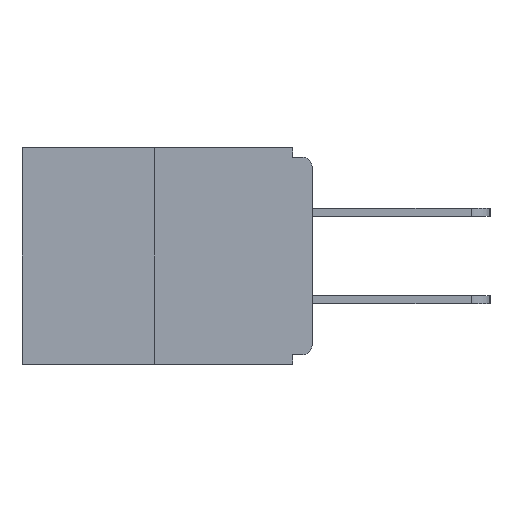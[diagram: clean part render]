
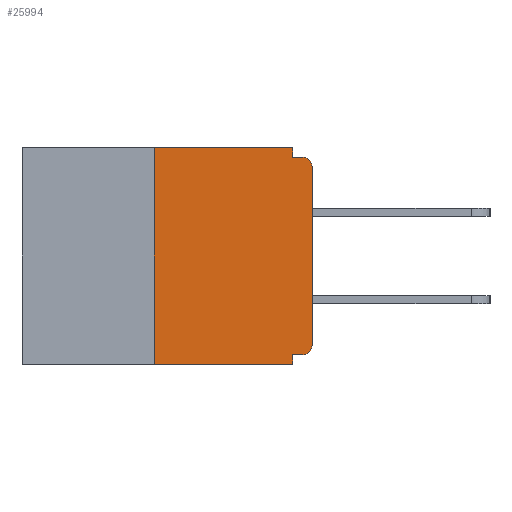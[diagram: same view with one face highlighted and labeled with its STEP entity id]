
A CAD part, left-side view. The second image highlights one B-rep face of the part: STEP entity #25994.
In plain terms, the highlighted planar face has unit normal (-1, 0, 0).
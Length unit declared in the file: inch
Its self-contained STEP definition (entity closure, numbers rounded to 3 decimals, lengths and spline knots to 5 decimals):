
#137 = DIRECTION ( 'NONE',  ( 0., 1., 0. ) ) ;
#1248 = LINE ( 'NONE', #21852, #16392 ) ;
#1658 = LINE ( 'NONE', #13782, #18388 ) ;
#2026 = LINE ( 'NONE', #14864, #24063 ) ;
#2213 = CARTESIAN_POINT ( 'NONE',  ( 0., 0., -0.328 ) ) ;
#2914 = DIRECTION ( 'NONE',  ( -1., 0., 0. ) ) ;
#3069 = DIRECTION ( 'NONE',  ( 0., 0., -1. ) ) ;
#3260 = CARTESIAN_POINT ( 'NONE',  ( 0., 0.031, -0.328 ) ) ;
#3447 = DIRECTION ( 'NONE',  ( 0., 0., -1. ) ) ;
#3623 = VECTOR ( 'NONE', #137, 39.37008 ) ;
#4881 = CARTESIAN_POINT ( 'NONE',  ( 0., 0.015, -0.313 ) ) ;
#4946 = CARTESIAN_POINT ( 'NONE',  ( 0., 0.46, 0. ) ) ;
#5291 = LINE ( 'NONE', #13303, #10782 ) ;
#5676 = CARTESIAN_POINT ( 'NONE',  ( 0., 0., -0.015 ) ) ;
#6066 = ORIENTED_EDGE ( 'NONE', *, *, #24553, .T. ) ;
#6385 = ORIENTED_EDGE ( 'NONE', *, *, #16559, .F. ) ;
#6531 = VERTEX_POINT ( 'NONE', #26326 ) ;
#6546 = ORIENTED_EDGE ( 'NONE', *, *, #11780, .F. ) ;
#6860 = EDGE_CURVE ( 'NONE', #15650, #23880, #1248, .T. ) ;
#7014 = ORIENTED_EDGE ( 'NONE', *, *, #19091, .T. ) ;
#7026 = VECTOR ( 'NONE', #22215, 39.37008 ) ;
#7319 = VERTEX_POINT ( 'NONE', #23950 ) ;
#7407 = PLANE ( 'NONE',  #8398 ) ;
#7681 = DIRECTION ( 'NONE',  ( 0., -1., 0. ) ) ;
#8398 = AXIS2_PLACEMENT_3D ( 'NONE', #9449, #11152, #25750 ) ;
#8469 = VERTEX_POINT ( 'NONE', #24242 ) ;
#8923 = VERTEX_POINT ( 'NONE', #3260 ) ;
#9086 = LINE ( 'NONE', #2213, #3623 ) ;
#9126 = DIRECTION ( 'NONE',  ( 0., 0., -1. ) ) ;
#9228 = ORIENTED_EDGE ( 'NONE', *, *, #6860, .T. ) ;
#9256 = LINE ( 'NONE', #5676, #7026 ) ;
#9421 = LINE ( 'NONE', #22024, #20637 ) ;
#9449 = CARTESIAN_POINT ( 'NONE',  ( 0., 0.46, 0. ) ) ;
#9699 = CIRCLE ( 'NONE', #12723, 0.015 ) ;
#9724 = VECTOR ( 'NONE', #21077, 39.37008 ) ;
#10782 = VECTOR ( 'NONE', #3069, 39.37008 ) ;
#11035 = CARTESIAN_POINT ( 'NONE',  ( 0., 0., -0.03 ) ) ;
#11149 = ORIENTED_EDGE ( 'NONE', *, *, #22864, .T. ) ;
#11152 = DIRECTION ( 'NONE',  ( 1., 0., 0. ) ) ;
#11780 = EDGE_CURVE ( 'NONE', #19613, #20787, #2026, .T. ) ;
#12723 = AXIS2_PLACEMENT_3D ( 'NONE', #14050, #15920, #3447 ) ;
#13303 = CARTESIAN_POINT ( 'NONE',  ( 0., 0.031, -0.343 ) ) ;
#13337 = VERTEX_POINT ( 'NONE', #16639 ) ;
#13609 = CARTESIAN_POINT ( 'NONE',  ( 0., 0.031, 0. ) ) ;
#13782 = CARTESIAN_POINT ( 'NONE',  ( 0., 0.031, 0. ) ) ;
#14050 = CARTESIAN_POINT ( 'NONE',  ( 0., 0.015, -0.03 ) ) ;
#14051 = ORIENTED_EDGE ( 'NONE', *, *, #15014, .F. ) ;
#14308 = ORIENTED_EDGE ( 'NONE', *, *, #18719, .F. ) ;
#14864 = CARTESIAN_POINT ( 'NONE',  ( 0., 0.25, 0. ) ) ;
#15014 = EDGE_CURVE ( 'NONE', #8923, #7319, #5291, .T. ) ;
#15650 = VERTEX_POINT ( 'NONE', #23675 ) ;
#15832 = ORIENTED_EDGE ( 'NONE', *, *, #21000, .F. ) ;
#15837 = ORIENTED_EDGE ( 'NONE', *, *, #25597, .F. ) ;
#15920 = DIRECTION ( 'NONE',  ( -1., 0., 0. ) ) ;
#16281 = CARTESIAN_POINT ( 'NONE',  ( 0., 0.25, 0. ) ) ;
#16392 = VECTOR ( 'NONE', #26255, 39.37008 ) ;
#16524 = EDGE_LOOP ( 'NONE', ( #14308, #6546, #6066, #14051, #6385, #11149, #9228, #7014, #15832, #15837 ) ) ;
#16559 = EDGE_CURVE ( 'NONE', #8469, #8923, #9086, .T. ) ;
#16639 = CARTESIAN_POINT ( 'NONE',  ( 0., 0.031, -0.015 ) ) ;
#18376 = DIRECTION ( 'NONE',  ( 0., 0., -1. ) ) ;
#18388 = VECTOR ( 'NONE', #18376, 39.37008 ) ;
#18719 = EDGE_CURVE ( 'NONE', #20787, #19657, #21829, .T. ) ;
#18951 = DIRECTION ( 'NONE',  ( 0., 0., 1. ) ) ;
#19091 = EDGE_CURVE ( 'NONE', #23880, #6531, #9699, .T. ) ;
#19613 = VERTEX_POINT ( 'NONE', #23762 ) ;
#19657 = VERTEX_POINT ( 'NONE', #13609 ) ;
#20637 = VECTOR ( 'NONE', #7681, 39.37008 ) ;
#20787 = VERTEX_POINT ( 'NONE', #16281 ) ;
#21000 = EDGE_CURVE ( 'NONE', #13337, #6531, #9256, .T. ) ;
#21077 = DIRECTION ( 'NONE',  ( 0., -1., 0. ) ) ;
#21829 = LINE ( 'NONE', #4946, #9724 ) ;
#21852 = CARTESIAN_POINT ( 'NONE',  ( 0., 0., 0. ) ) ;
#22024 = CARTESIAN_POINT ( 'NONE',  ( 0., 0.46, -0.343 ) ) ;
#22215 = DIRECTION ( 'NONE',  ( 0., -1., 0. ) ) ;
#22864 = EDGE_CURVE ( 'NONE', #8469, #15650, #22955, .T. ) ;
#22955 = CIRCLE ( 'NONE', #25890, 0.015 ) ;
#23675 = CARTESIAN_POINT ( 'NONE',  ( 0., 0., -0.313 ) ) ;
#23762 = CARTESIAN_POINT ( 'NONE',  ( 0., 0.25, -0.343 ) ) ;
#23880 = VERTEX_POINT ( 'NONE', #11035 ) ;
#23950 = CARTESIAN_POINT ( 'NONE',  ( 0., 0.031, -0.343 ) ) ;
#24063 = VECTOR ( 'NONE', #18951, 39.37008 ) ;
#24242 = CARTESIAN_POINT ( 'NONE',  ( 0., 0.015, -0.328 ) ) ;
#24553 = EDGE_CURVE ( 'NONE', #19613, #7319, #9421, .T. ) ;
#24700 = FACE_OUTER_BOUND ( 'NONE', #16524, .T. ) ;
#25597 = EDGE_CURVE ( 'NONE', #19657, #13337, #1658, .T. ) ;
#25750 = DIRECTION ( 'NONE',  ( 0., 0., -1. ) ) ;
#25890 = AXIS2_PLACEMENT_3D ( 'NONE', #4881, #2914, #9126 ) ;
#25994 = ADVANCED_FACE ( 'NONE', ( #24700 ), #7407, .F. ) ;
#26255 = DIRECTION ( 'NONE',  ( 0., 0., 1. ) ) ;
#26326 = CARTESIAN_POINT ( 'NONE',  ( 0., 0.015, -0.015 ) ) ;
